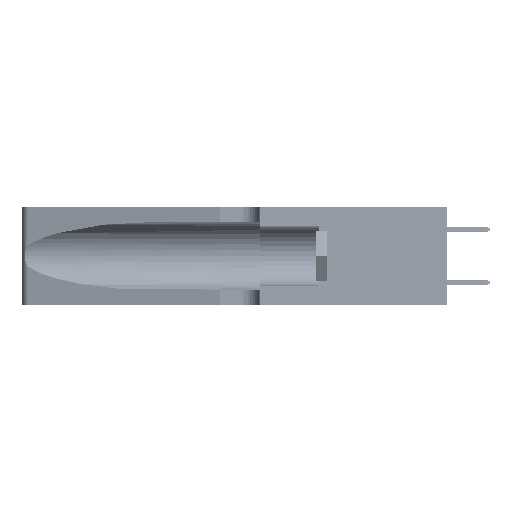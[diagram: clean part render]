
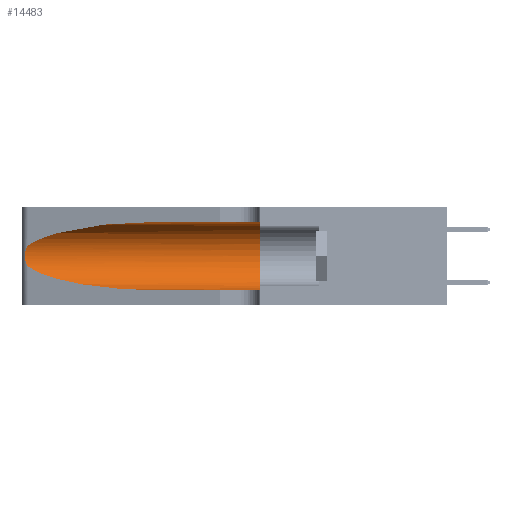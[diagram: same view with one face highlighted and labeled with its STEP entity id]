
A CAD part, left-side view. The second image highlights one B-rep face of the part: STEP entity #14483.
In plain terms, the highlighted cylindrical face has radius 3.308 mm (diameter 6.617 mm), a partial arc.
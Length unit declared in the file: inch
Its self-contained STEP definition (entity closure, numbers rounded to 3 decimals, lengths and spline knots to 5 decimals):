
#1935 = EDGE_CURVE ( 'NONE', #30577, #17108, #49738, .T. ) ;
#2543 = DIRECTION ( 'NONE',  ( 0., 0., 1. ) ) ;
#2626 = LINE ( 'NONE', #5401, #25110 ) ;
#2656 = CARTESIAN_POINT ( 'NONE',  ( 0.2373, 1.15595, 0.28018 ) ) ;
#3051 = CARTESIAN_POINT ( 'NONE',  ( 0.1305, 0.72297, 0.05475 ) ) ;
#4390 = EDGE_CURVE ( 'NONE', #32589, #34924, #7108, .T. ) ;
#5401 = CARTESIAN_POINT ( 'NONE',  ( 0.1305, 1.61858, 0.31525 ) ) ;
#5688 = DIRECTION ( 'NONE',  ( 0., -1., 0. ) ) ;
#6984 = CARTESIAN_POINT ( 'NONE',  ( 0.18966, 0.96281, 0.31525 ) ) ;
#7108 = LINE ( 'NONE', #47312, #7161 ) ;
#7161 = VECTOR ( 'NONE', #23533, 39.37008 ) ;
#7386 = CARTESIAN_POINT ( 'NONE',  ( 0.26017, 1.23833, 0.17102 ) ) ;
#9000 = VERTEX_POINT ( 'NONE', #26196 ) ;
#10031 = CARTESIAN_POINT ( 'NONE',  ( 0.1305, 1.61858, 0.185 ) ) ;
#11695 = ORIENTED_EDGE ( 'NONE', *, *, #16610, .F. ) ;
#11699 = ORIENTED_EDGE ( 'NONE', *, *, #20063, .T. ) ;
#12766 = EDGE_CURVE ( 'NONE', #18619, #9000, #2626, .T. ) ;
#13514 = DIRECTION ( 'NONE',  ( 0., 0., -1. ) ) ;
#14357 = ORIENTED_EDGE ( 'NONE', *, *, #12766, .F. ) ;
#14483 = ADVANCED_FACE ( 'NONE', ( #44621 ), #28521, .F. ) ;
#15891 = CARTESIAN_POINT ( 'NONE',  ( 0.1305, 0.72297, 0.31525 ) ) ;
#16285 = CARTESIAN_POINT ( 'NONE',  ( 0.25555, 1.22993, 0.14849 ) ) ;
#16610 = EDGE_CURVE ( 'NONE', #9000, #34924, #48098, .T. ) ;
#16633 = CARTESIAN_POINT ( 'NONE',  ( 0.25487, 1.22718, 0.14631 ) ) ;
#17108 = VERTEX_POINT ( 'NONE', #45867 ) ;
#17286 = EDGE_CURVE ( 'NONE', #18619, #30577, #41461, .T. ) ;
#18619 = VERTEX_POINT ( 'NONE', #15891 ) ;
#19451 = CARTESIAN_POINT ( 'NONE',  ( 0.18966, 0.96281, 0.05475 ) ) ;
#20063 = EDGE_CURVE ( 'NONE', #17108, #32589, #40514, .T. ) ;
#20514 = CARTESIAN_POINT ( 'NONE',  ( 0.25639, 1.23186, 0.15144 ) ) ;
#22105 = CARTESIAN_POINT ( 'NONE',  ( 0.1305, 0.35, 0.185 ) ) ;
#23512 = CARTESIAN_POINT ( 'NONE',  ( 0.25787, 1.23484, 0.2124 ) ) ;
#23533 = DIRECTION ( 'NONE',  ( 0., -1., 0. ) ) ;
#23839 = CARTESIAN_POINT ( 'NONE',  ( 0.26018, 1.23835, 0.19895 ) ) ;
#25110 = VECTOR ( 'NONE', #28931, 39.37008 ) ;
#26183 = EDGE_LOOP ( 'NONE', ( #29913, #31261, #11699, #29860, #11695, #14357 ) ) ;
#26196 = CARTESIAN_POINT ( 'NONE',  ( 0.1305, 0.35, 0.31525 ) ) ;
#28011 = CARTESIAN_POINT ( 'NONE',  ( 0.25639, 1.23184, 0.21858 ) ) ;
#28521 = CYLINDRICAL_SURFACE ( 'NONE', #40089, 0.13025 ) ;
#28931 = DIRECTION ( 'NONE',  ( 0., -1., 0. ) ) ;
#29860 = ORIENTED_EDGE ( 'NONE', *, *, #4390, .T. ) ;
#29913 = ORIENTED_EDGE ( 'NONE', *, *, #17286, .T. ) ;
#30577 = VERTEX_POINT ( 'NONE', #31272 ) ;
#31111 = CARTESIAN_POINT ( 'NONE',  ( 0.25555, 1.22994, 0.2215 ) ) ;
#31239 = CARTESIAN_POINT ( 'NONE',  ( 0.25487, 1.22718, 0.14631 ) ) ;
#31261 = ORIENTED_EDGE ( 'NONE', *, *, #1935, .T. ) ;
#31272 = CARTESIAN_POINT ( 'NONE',  ( 0.25487, 1.22718, 0.22369 ) ) ;
#31827 = CARTESIAN_POINT ( 'NONE',  ( 0.26075, 1.23896, 0.19203 ) ) ;
#32589 = VERTEX_POINT ( 'NONE', #3051 ) ;
#34924 = VERTEX_POINT ( 'NONE', #37880 ) ;
#35644 = CARTESIAN_POINT ( 'NONE',  ( 0.1305, 0.72297, 0.05475 ) ) ;
#36002 = CARTESIAN_POINT ( 'NONE',  ( 0.25856, 1.23593, 0.16098 ) ) ;
#37880 = CARTESIAN_POINT ( 'NONE',  ( 0.1305, 0.35, 0.05475 ) ) ;
#38763 = CARTESIAN_POINT ( 'NONE',  ( 0.25487, 1.22718, 0.22369 ) ) ;
#40089 = AXIS2_PLACEMENT_3D ( 'NONE', #10031, #5688, #13514 ) ;
#40159 = CARTESIAN_POINT ( 'NONE',  ( 0.25789, 1.23486, 0.15765 ) ) ;
#40514 =( BOUNDED_CURVE ( )  B_SPLINE_CURVE ( 3, ( #31239, #43627, #19451, #35644 ),
 .UNSPECIFIED., .F., .F. ) 
 B_SPLINE_CURVE_WITH_KNOTS ( ( 4, 4 ),
 ( 3.44316, 4.71239 ),
 .UNSPECIFIED. ) 
 CURVE ( )  GEOMETRIC_REPRESENTATION_ITEM ( )  RATIONAL_B_SPLINE_CURVE ( ( 1., 0.87, 0.87, 1. ) ) 
 REPRESENTATION_ITEM ( '' )  );
#41090 = AXIS2_PLACEMENT_3D ( 'NONE', #22105, #50402, #2543 ) ;
#41461 =( BOUNDED_CURVE ( )  B_SPLINE_CURVE ( 3, ( #50337, #6984, #2656, #50515 ),
 .UNSPECIFIED., .F., .F. ) 
 B_SPLINE_CURVE_WITH_KNOTS ( ( 4, 4 ),
 ( 1.5708, 2.84003 ),
 .UNSPECIFIED. ) 
 CURVE ( )  GEOMETRIC_REPRESENTATION_ITEM ( )  RATIONAL_B_SPLINE_CURVE ( ( 1., 0.87, 0.87, 1. ) ) 
 REPRESENTATION_ITEM ( '' )  );
#43627 = CARTESIAN_POINT ( 'NONE',  ( 0.2373, 1.15595, 0.08982 ) ) ;
#44621 = FACE_OUTER_BOUND ( 'NONE', #26183, .T. ) ;
#45867 = CARTESIAN_POINT ( 'NONE',  ( 0.25487, 1.22718, 0.14631 ) ) ;
#47109 = CARTESIAN_POINT ( 'NONE',  ( 0.26075, 1.23896, 0.178 ) ) ;
#47312 = CARTESIAN_POINT ( 'NONE',  ( 0.1305, 1.61858, 0.05475 ) ) ;
#48098 = CIRCLE ( 'NONE', #41090, 0.13025 ) ;
#49738 = B_SPLINE_CURVE_WITH_KNOTS ( 'NONE', 3,
 ( #38763, #31111, #28011, #23512, #51473, #23839, #31827, #47109, #7386, #36002, #40159, #20514, #16285, #16633 ),
 .UNSPECIFIED., .F., .F.,
 ( 4, 2, 2, 2, 2, 2, 4 ),
 ( 0., 0.00027, 0.00053, 0.00107, 0.0016, 0.00187, 0.00214 ),
 .UNSPECIFIED. ) ;
#50337 = CARTESIAN_POINT ( 'NONE',  ( 0.1305, 0.72297, 0.31525 ) ) ;
#50402 = DIRECTION ( 'NONE',  ( 0., 1., 0. ) ) ;
#50515 = CARTESIAN_POINT ( 'NONE',  ( 0.25487, 1.22718, 0.22369 ) ) ;
#51473 = CARTESIAN_POINT ( 'NONE',  ( 0.25854, 1.2359, 0.20912 ) ) ;
